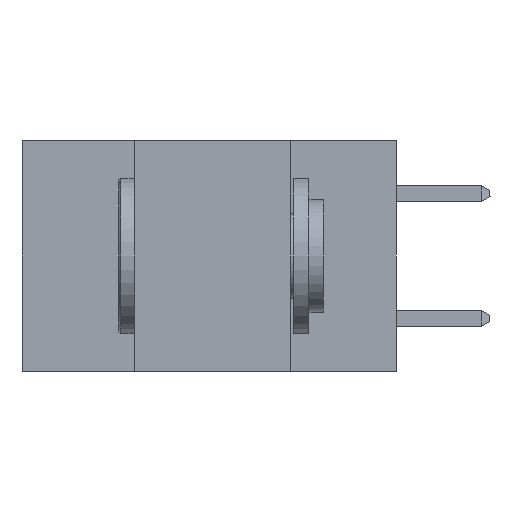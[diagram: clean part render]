
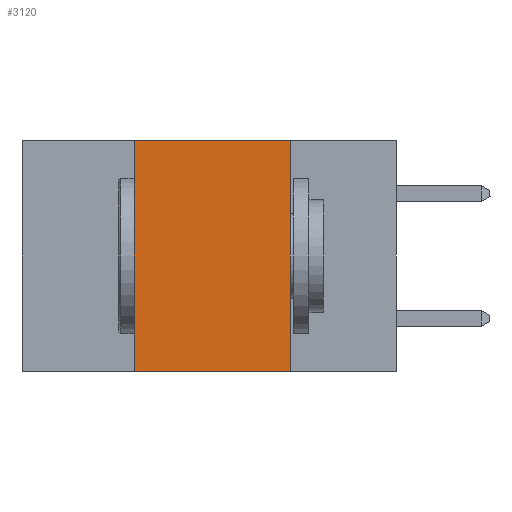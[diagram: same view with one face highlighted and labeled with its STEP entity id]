
A CAD part, left-side view. The second image highlights one B-rep face of the part: STEP entity #3120.
In plain terms, the highlighted planar face has unit normal (-1, 0, 0).
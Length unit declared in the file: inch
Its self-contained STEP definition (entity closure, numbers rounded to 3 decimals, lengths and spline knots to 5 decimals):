
#86 = DIRECTION ( 'NONE',  ( 0., -1., 0. ) ) ;
#492 = ORIENTED_EDGE ( 'NONE', *, *, #7393, .F. ) ;
#806 = ORIENTED_EDGE ( 'NONE', *, *, #10736, .F. ) ;
#894 = LINE ( 'NONE', #12181, #4382 ) ;
#2936 = EDGE_LOOP ( 'NONE', ( #492, #20974, #806, #10305 ) ) ;
#3120 = ADVANCED_FACE ( 'NONE', ( #10885 ), #10525, .F. ) ;
#3191 = LINE ( 'NONE', #20252, #19923 ) ;
#3411 = LINE ( 'NONE', #11904, #16187 ) ;
#4275 = CARTESIAN_POINT ( 'NONE',  ( 0., 0.6, -0.37 ) ) ;
#4382 = VECTOR ( 'NONE', #5556, 39.37008 ) ;
#4972 = VECTOR ( 'NONE', #5957, 39.37008 ) ;
#5556 = DIRECTION ( 'NONE',  ( 0., 0., -1. ) ) ;
#5957 = DIRECTION ( 'NONE',  ( 0., -1., 0. ) ) ;
#6781 = CARTESIAN_POINT ( 'NONE',  ( 0., 0.17, -0.37 ) ) ;
#7393 = EDGE_CURVE ( 'NONE', #20120, #14396, #894, .T. ) ;
#8189 = CARTESIAN_POINT ( 'NONE',  ( 0., 0.42, -0.37 ) ) ;
#10305 = ORIENTED_EDGE ( 'NONE', *, *, #14044, .T. ) ;
#10525 = PLANE ( 'NONE',  #18340 ) ;
#10542 = CARTESIAN_POINT ( 'NONE',  ( 0., 0.6, 0. ) ) ;
#10736 = EDGE_CURVE ( 'NONE', #11801, #15545, #3191, .T. ) ;
#10885 = FACE_OUTER_BOUND ( 'NONE', #2936, .T. ) ;
#11801 = VERTEX_POINT ( 'NONE', #8189 ) ;
#11904 = CARTESIAN_POINT ( 'NONE',  ( 0., 0.6, 0. ) ) ;
#12181 = CARTESIAN_POINT ( 'NONE',  ( 0., 0.17, 0. ) ) ;
#14044 = EDGE_CURVE ( 'NONE', #11801, #14396, #18256, .T. ) ;
#14396 = VERTEX_POINT ( 'NONE', #6781 ) ;
#15274 = DIRECTION ( 'NONE',  ( 0., 0., 1. ) ) ;
#15545 = VERTEX_POINT ( 'NONE', #18207 ) ;
#15637 = DIRECTION ( 'NONE',  ( 1., 0., 0. ) ) ;
#15712 = CARTESIAN_POINT ( 'NONE',  ( 0., 0.17, 0. ) ) ;
#16187 = VECTOR ( 'NONE', #86, 39.37008 ) ;
#18207 = CARTESIAN_POINT ( 'NONE',  ( 0., 0.42, 0. ) ) ;
#18256 = LINE ( 'NONE', #4275, #4972 ) ;
#18340 = AXIS2_PLACEMENT_3D ( 'NONE', #10542, #15637, #20440 ) ;
#19923 = VECTOR ( 'NONE', #15274, 39.37008 ) ;
#20120 = VERTEX_POINT ( 'NONE', #15712 ) ;
#20252 = CARTESIAN_POINT ( 'NONE',  ( 0., 0.42, 0. ) ) ;
#20440 = DIRECTION ( 'NONE',  ( 0., 0., -1. ) ) ;
#20974 = ORIENTED_EDGE ( 'NONE', *, *, #21450, .F. ) ;
#21450 = EDGE_CURVE ( 'NONE', #15545, #20120, #3411, .T. ) ;
